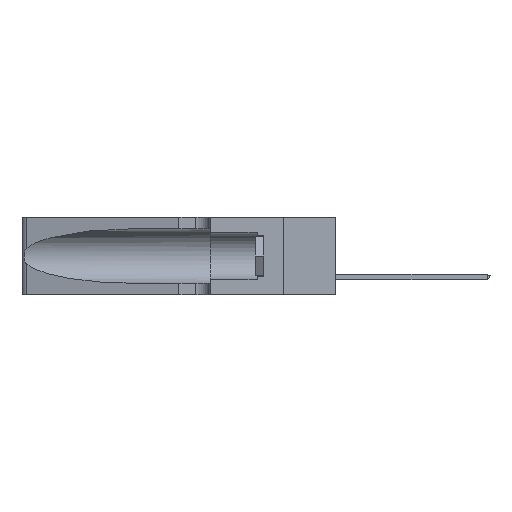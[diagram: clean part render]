
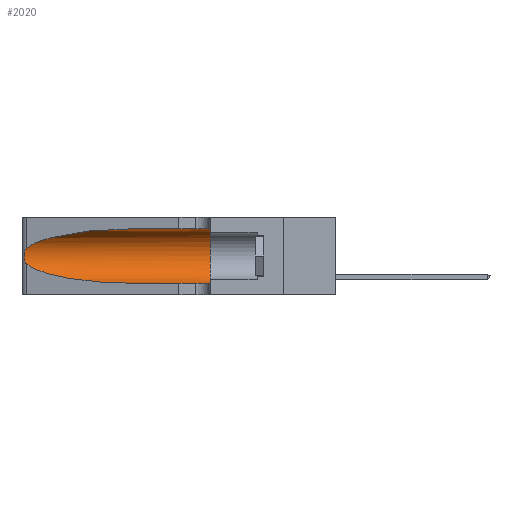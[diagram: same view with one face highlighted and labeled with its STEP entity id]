
A CAD part, left-side view. The second image highlights one B-rep face of the part: STEP entity #2020.
In plain terms, the highlighted cylindrical face has radius 3.308 mm (diameter 6.617 mm), a partial arc.
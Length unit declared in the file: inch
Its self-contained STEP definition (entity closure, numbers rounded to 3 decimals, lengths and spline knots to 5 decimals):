
#924 = DIRECTION ( 'NONE',  ( 0., -1., 0. ) ) ;
#1404 = CARTESIAN_POINT ( 'NONE',  ( 0.25854, 1.2359, 0.20912 ) ) ;
#1493 = CARTESIAN_POINT ( 'NONE',  ( 0.25787, 1.23484, 0.2124 ) ) ;
#2020 = ADVANCED_FACE ( 'NONE', ( #4869 ), #26374, .F. ) ;
#2225 = VERTEX_POINT ( 'NONE', #18983 ) ;
#2672 = CARTESIAN_POINT ( 'NONE',  ( 0.1305, 0.35, 0.185 ) ) ;
#3018 = CARTESIAN_POINT ( 'NONE',  ( 0.18966, 0.96281, 0.05475 ) ) ;
#3398 = CARTESIAN_POINT ( 'NONE',  ( 0.25856, 1.23593, 0.16098 ) ) ;
#3464 = CARTESIAN_POINT ( 'NONE',  ( 0.1305, 0.72297, 0.31525 ) ) ;
#3593 = CARTESIAN_POINT ( 'NONE',  ( 0.26018, 1.23835, 0.19895 ) ) ;
#3872 = VECTOR ( 'NONE', #4847, 39.37008 ) ;
#4542 = CARTESIAN_POINT ( 'NONE',  ( 0.1305, 0.72297, 0.31525 ) ) ;
#4753 = VERTEX_POINT ( 'NONE', #17551 ) ;
#4847 = DIRECTION ( 'NONE',  ( 0., -1., 0. ) ) ;
#4869 = FACE_OUTER_BOUND ( 'NONE', #14350, .T. ) ;
#5063 = CARTESIAN_POINT ( 'NONE',  ( 0.1305, 0.35, 0.31525 ) ) ;
#5092 = VECTOR ( 'NONE', #924, 39.37008 ) ;
#5125 = CARTESIAN_POINT ( 'NONE',  ( 0.2373, 1.15595, 0.08982 ) ) ;
#5230 = CARTESIAN_POINT ( 'NONE',  ( 0.1305, 0.72297, 0.05475 ) ) ;
#5772 = EDGE_CURVE ( 'NONE', #4753, #25235, #17327, .T. ) ;
#6627 = DIRECTION ( 'NONE',  ( 0., 1., 0. ) ) ;
#6711 = ORIENTED_EDGE ( 'NONE', *, *, #22258, .T. ) ;
#6733 = EDGE_CURVE ( 'NONE', #12603, #23029, #13259, .T. ) ;
#7309 = CARTESIAN_POINT ( 'NONE',  ( 0.2373, 1.15595, 0.28018 ) ) ;
#7636 = CARTESIAN_POINT ( 'NONE',  ( 0.25639, 1.23186, 0.15144 ) ) ;
#7824 = DIRECTION ( 'NONE',  ( 0., -1., 0. ) ) ;
#7989 = CARTESIAN_POINT ( 'NONE',  ( 0.25555, 1.22994, 0.2215 ) ) ;
#9411 = VERTEX_POINT ( 'NONE', #17208 ) ;
#9599 = CIRCLE ( 'NONE', #19723, 0.13025 ) ;
#9902 = CARTESIAN_POINT ( 'NONE',  ( 0.25487, 1.22718, 0.14631 ) ) ;
#10888 = CARTESIAN_POINT ( 'NONE',  ( 0.1305, 1.61858, 0.05475 ) ) ;
#10979 = DIRECTION ( 'NONE',  ( 0., 0., 1. ) ) ;
#11139 = ORIENTED_EDGE ( 'NONE', *, *, #23369, .T. ) ;
#11725 = CARTESIAN_POINT ( 'NONE',  ( 0.26075, 1.23896, 0.178 ) ) ;
#11829 = CARTESIAN_POINT ( 'NONE',  ( 0.1305, 1.61858, 0.185 ) ) ;
#11870 = CARTESIAN_POINT ( 'NONE',  ( 0.1305, 0.72297, 0.05475 ) ) ;
#12603 = VERTEX_POINT ( 'NONE', #3464 ) ;
#12923 = ORIENTED_EDGE ( 'NONE', *, *, #14367, .F. ) ;
#13259 = LINE ( 'NONE', #19417, #5092 ) ;
#13849 = AXIS2_PLACEMENT_3D ( 'NONE', #11829, #7824, #14081 ) ;
#13884 = CARTESIAN_POINT ( 'NONE',  ( 0.26017, 1.23833, 0.17102 ) ) ;
#14081 = DIRECTION ( 'NONE',  ( 0., 0., -1. ) ) ;
#14155 = CARTESIAN_POINT ( 'NONE',  ( 0.25789, 1.23486, 0.15765 ) ) ;
#14350 = EDGE_LOOP ( 'NONE', ( #6711, #11139, #14950, #17845, #12923, #26235 ) ) ;
#14367 = EDGE_CURVE ( 'NONE', #23029, #2225, #9599, .T. ) ;
#14950 = ORIENTED_EDGE ( 'NONE', *, *, #5772, .T. ) ;
#15393 = CARTESIAN_POINT ( 'NONE',  ( 0.25487, 1.22718, 0.22369 ) ) ;
#15993 = CARTESIAN_POINT ( 'NONE',  ( 0.25555, 1.22993, 0.14849 ) ) ;
#17208 = CARTESIAN_POINT ( 'NONE',  ( 0.25487, 1.22718, 0.22369 ) ) ;
#17327 =( BOUNDED_CURVE ( )  B_SPLINE_CURVE ( 3, ( #22045, #5125, #3018, #11870 ),
 .UNSPECIFIED., .F., .F. ) 
 B_SPLINE_CURVE_WITH_KNOTS ( ( 4, 4 ),
 ( 3.44316, 4.71239 ),
 .UNSPECIFIED. ) 
 CURVE ( )  GEOMETRIC_REPRESENTATION_ITEM ( )  RATIONAL_B_SPLINE_CURVE ( ( 1., 0.87, 0.87, 1. ) ) 
 REPRESENTATION_ITEM ( '' )  );
#17551 = CARTESIAN_POINT ( 'NONE',  ( 0.25487, 1.22718, 0.14631 ) ) ;
#17845 = ORIENTED_EDGE ( 'NONE', *, *, #25720, .T. ) ;
#18983 = CARTESIAN_POINT ( 'NONE',  ( 0.1305, 0.35, 0.05475 ) ) ;
#19417 = CARTESIAN_POINT ( 'NONE',  ( 0.1305, 1.61858, 0.31525 ) ) ;
#19723 = AXIS2_PLACEMENT_3D ( 'NONE', #2672, #6627, #10979 ) ;
#20618 = B_SPLINE_CURVE_WITH_KNOTS ( 'NONE', 3,
 ( #24425, #7989, #26626, #1493, #1404, #3593, #24529, #11725, #13884, #3398, #14155, #7636, #15993, #9902 ),
 .UNSPECIFIED., .F., .F.,
 ( 4, 2, 2, 2, 2, 2, 4 ),
 ( 0., 0.00027, 0.00053, 0.00107, 0.0016, 0.00187, 0.00214 ),
 .UNSPECIFIED. ) ;
#21138 =( BOUNDED_CURVE ( )  B_SPLINE_CURVE ( 3, ( #4542, #21383, #7309, #15393 ),
 .UNSPECIFIED., .F., .T. ) 
 B_SPLINE_CURVE_WITH_KNOTS ( ( 4, 4 ),
 ( 1.5708, 2.84003 ),
 .UNSPECIFIED. ) 
 CURVE ( )  GEOMETRIC_REPRESENTATION_ITEM ( )  RATIONAL_B_SPLINE_CURVE ( ( 1., 0.87, 0.87, 1. ) ) 
 REPRESENTATION_ITEM ( '' )  );
#21383 = CARTESIAN_POINT ( 'NONE',  ( 0.18966, 0.96281, 0.31525 ) ) ;
#22045 = CARTESIAN_POINT ( 'NONE',  ( 0.25487, 1.22718, 0.14631 ) ) ;
#22258 = EDGE_CURVE ( 'NONE', #12603, #9411, #21138, .T. ) ;
#23029 = VERTEX_POINT ( 'NONE', #5063 ) ;
#23369 = EDGE_CURVE ( 'NONE', #9411, #4753, #20618, .T. ) ;
#24425 = CARTESIAN_POINT ( 'NONE',  ( 0.25487, 1.22718, 0.22369 ) ) ;
#24529 = CARTESIAN_POINT ( 'NONE',  ( 0.26075, 1.23896, 0.19203 ) ) ;
#25235 = VERTEX_POINT ( 'NONE', #5230 ) ;
#25720 = EDGE_CURVE ( 'NONE', #25235, #2225, #26045, .T. ) ;
#26045 = LINE ( 'NONE', #10888, #3872 ) ;
#26235 = ORIENTED_EDGE ( 'NONE', *, *, #6733, .F. ) ;
#26374 = CYLINDRICAL_SURFACE ( 'NONE', #13849, 0.13025 ) ;
#26626 = CARTESIAN_POINT ( 'NONE',  ( 0.25639, 1.23184, 0.21858 ) ) ;
